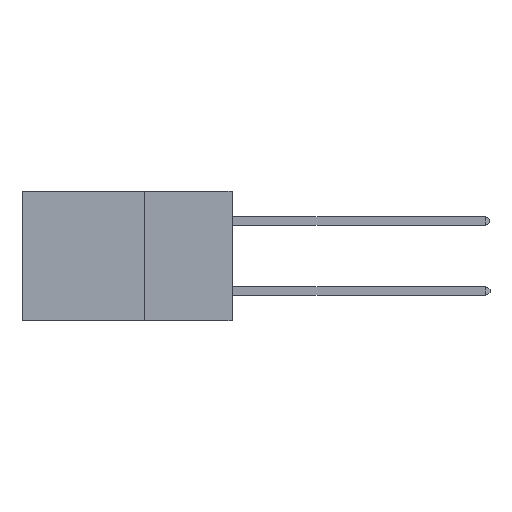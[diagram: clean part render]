
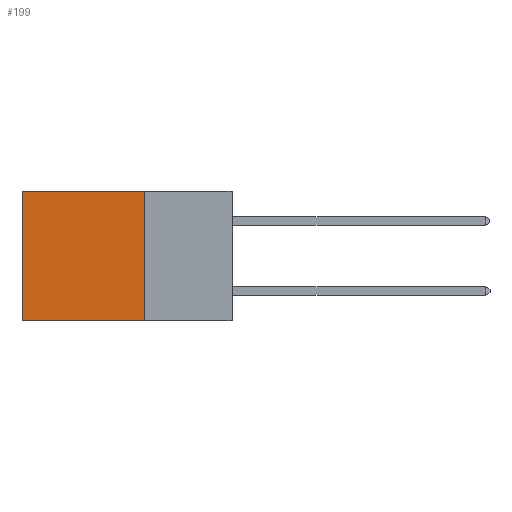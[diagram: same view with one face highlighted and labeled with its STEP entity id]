
A CAD part, left-side view. The second image highlights one B-rep face of the part: STEP entity #199.
In plain terms, the highlighted planar face has unit normal (-1, 0, 0).
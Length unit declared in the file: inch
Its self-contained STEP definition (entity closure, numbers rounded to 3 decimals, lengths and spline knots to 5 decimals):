
#31 = LINE ( 'NONE', #8377, #4250 ) ;
#199 = ADVANCED_FACE ( 'NONE', ( #2976 ), #13397, .F. ) ;
#349 = DIRECTION ( 'NONE',  ( 0., 1., 0. ) ) ;
#436 = DIRECTION ( 'NONE',  ( 0., 1., 0. ) ) ;
#496 = VECTOR ( 'NONE', #349, 39.37008 ) ;
#1127 = VERTEX_POINT ( 'NONE', #22356 ) ;
#1802 = ORIENTED_EDGE ( 'NONE', *, *, #20843, .F. ) ;
#2805 = CARTESIAN_POINT ( 'NONE',  ( 0.2875, 0.6, 0. ) ) ;
#2976 = FACE_OUTER_BOUND ( 'NONE', #22572, .T. ) ;
#3011 = LINE ( 'NONE', #14630, #7236 ) ;
#4122 = DIRECTION ( 'NONE',  ( 0., 0., -1. ) ) ;
#4250 = VECTOR ( 'NONE', #4752, 39.37008 ) ;
#4622 = EDGE_CURVE ( 'NONE', #1127, #8063, #3011, .T. ) ;
#4752 = DIRECTION ( 'NONE',  ( 0., 0., -1. ) ) ;
#7236 = VECTOR ( 'NONE', #4122, 39.37008 ) ;
#7453 = CARTESIAN_POINT ( 'NONE',  ( 0.2875, 0.25, 0. ) ) ;
#7595 = CARTESIAN_POINT ( 'NONE',  ( 0.2875, 0.25, 0. ) ) ;
#7984 = EDGE_CURVE ( 'NONE', #1127, #18598, #9890, .T. ) ;
#8063 = VERTEX_POINT ( 'NONE', #9623 ) ;
#8227 = EDGE_CURVE ( 'NONE', #18598, #17877, #31, .T. ) ;
#8377 = CARTESIAN_POINT ( 'NONE',  ( 0.2875, 0.6, 0. ) ) ;
#8773 = ORIENTED_EDGE ( 'NONE', *, *, #4622, .F. ) ;
#9623 = CARTESIAN_POINT ( 'NONE',  ( 0.2875, 0.25, -0.37 ) ) ;
#9890 = LINE ( 'NONE', #7595, #21426 ) ;
#11098 = DIRECTION ( 'NONE',  ( 1., 0., 0. ) ) ;
#13184 = CARTESIAN_POINT ( 'NONE',  ( 0.2875, 0.6, -0.37 ) ) ;
#13397 = PLANE ( 'NONE',  #19264 ) ;
#14630 = CARTESIAN_POINT ( 'NONE',  ( 0.2875, 0.25, 0. ) ) ;
#17357 = ORIENTED_EDGE ( 'NONE', *, *, #7984, .T. ) ;
#17782 = ORIENTED_EDGE ( 'NONE', *, *, #8227, .T. ) ;
#17877 = VERTEX_POINT ( 'NONE', #13184 ) ;
#18598 = VERTEX_POINT ( 'NONE', #2805 ) ;
#18782 = LINE ( 'NONE', #21595, #496 ) ;
#19057 = DIRECTION ( 'NONE',  ( 0., 0., -1. ) ) ;
#19264 = AXIS2_PLACEMENT_3D ( 'NONE', #7453, #11098, #19057 ) ;
#20843 = EDGE_CURVE ( 'NONE', #8063, #17877, #18782, .T. ) ;
#21426 = VECTOR ( 'NONE', #436, 39.37008 ) ;
#21595 = CARTESIAN_POINT ( 'NONE',  ( 0.2875, 0.25, -0.37 ) ) ;
#22356 = CARTESIAN_POINT ( 'NONE',  ( 0.2875, 0.25, 0. ) ) ;
#22572 = EDGE_LOOP ( 'NONE', ( #17782, #1802, #8773, #17357 ) ) ;
